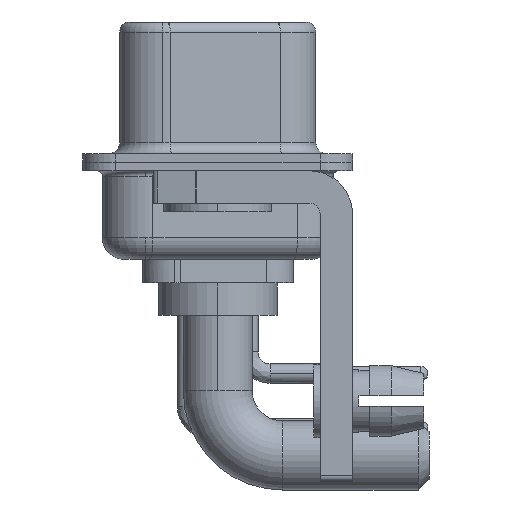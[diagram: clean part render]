
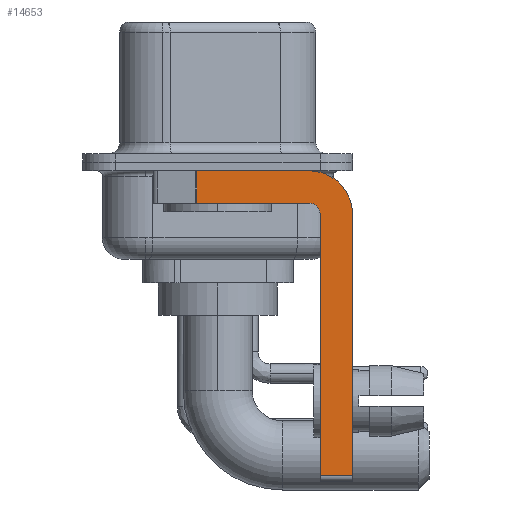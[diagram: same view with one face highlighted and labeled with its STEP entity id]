
A CAD part, left-side view. The second image highlights one B-rep face of the part: STEP entity #14653.
In plain terms, the highlighted planar face has unit normal (-1, 0, 0).
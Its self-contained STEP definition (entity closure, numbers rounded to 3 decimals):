
#846 = DIRECTION ( 'NONE',  ( 0., 0., -1. ) ) ;
#944 = EDGE_CURVE ( 'NONE', #23648, #19559, #24947, .T. ) ;
#1012 = VERTEX_POINT ( 'NONE', #1270 ) ;
#1270 = CARTESIAN_POINT ( 'NONE',  ( -2.9, -4.25, -0.4 ) ) ;
#1272 = LINE ( 'NONE', #3926, #5003 ) ;
#1379 = CARTESIAN_POINT ( 'NONE',  ( -2.9, 3., -0.4 ) ) ;
#2157 = VECTOR ( 'NONE', #846, 1000. ) ;
#2641 = VECTOR ( 'NONE', #6924, 1000. ) ;
#2652 = ORIENTED_EDGE ( 'NONE', *, *, #17154, .F. ) ;
#3075 = AXIS2_PLACEMENT_3D ( 'NONE', #25043, #11268, #29862 ) ;
#3139 = DIRECTION ( 'NONE',  ( 0., 0., -1. ) ) ;
#3926 = CARTESIAN_POINT ( 'NONE',  ( -2.9, -4.75, -14.8 ) ) ;
#4272 = EDGE_CURVE ( 'NONE', #19559, #4273, #13885, .T. ) ;
#4273 = VERTEX_POINT ( 'NONE', #29976 ) ;
#4449 = AXIS2_PLACEMENT_3D ( 'NONE', #12879, #17130, #22141 ) ;
#5003 = VECTOR ( 'NONE', #8788, 1000. ) ;
#5857 = CARTESIAN_POINT ( 'NONE',  ( -2.9, -4.25, -14.55 ) ) ;
#5903 = EDGE_CURVE ( 'NONE', #22991, #4273, #27285, .T. ) ;
#6349 = EDGE_CURVE ( 'NONE', #22991, #1012, #22850, .T. ) ;
#6483 = DIRECTION ( 'NONE',  ( 1., 0., 0. ) ) ;
#6924 = DIRECTION ( 'NONE',  ( 0., -1., 0. ) ) ;
#7840 = CIRCLE ( 'NONE', #25843, 2. ) ;
#8675 = CARTESIAN_POINT ( 'NONE',  ( -2.9, -6.25, -2.4 ) ) ;
#8788 = DIRECTION ( 'NONE',  ( 0., 0., 1. ) ) ;
#9100 = EDGE_LOOP ( 'NONE', ( #12794, #27243, #21199, #10554, #2652, #26335, #9128, #10559 ) ) ;
#9128 = ORIENTED_EDGE ( 'NONE', *, *, #29358, .F. ) ;
#9729 = LINE ( 'NONE', #28971, #23791 ) ;
#10554 = ORIENTED_EDGE ( 'NONE', *, *, #944, .F. ) ;
#10559 = ORIENTED_EDGE ( 'NONE', *, *, #30675, .F. ) ;
#11067 = CARTESIAN_POINT ( 'NONE',  ( -2.9, -4.25, -1.9 ) ) ;
#11268 = DIRECTION ( 'NONE',  ( 1., 0., 0. ) ) ;
#12794 = ORIENTED_EDGE ( 'NONE', *, *, #6349, .F. ) ;
#12879 = CARTESIAN_POINT ( 'NONE',  ( -2.9, -4.25, -2.4 ) ) ;
#13539 = CARTESIAN_POINT ( 'NONE',  ( -2.9, -4.75, -2.4 ) ) ;
#13574 = DIRECTION ( 'NONE',  ( 0., 1., 0. ) ) ;
#13885 = LINE ( 'NONE', #11067, #28058 ) ;
#14653 = ADVANCED_FACE ( 'NONE', ( #23173 ), #17850, .F. ) ;
#15641 = DIRECTION ( 'NONE',  ( 0., -1., 0. ) ) ;
#15690 = VECTOR ( 'NONE', #15641, 1000. ) ;
#17130 = DIRECTION ( 'NONE',  ( -1., 0., 0. ) ) ;
#17154 = EDGE_CURVE ( 'NONE', #22116, #23648, #1272, .T. ) ;
#17850 = PLANE ( 'NONE',  #3075 ) ;
#18411 = CARTESIAN_POINT ( 'NONE',  ( -2.9, -4.25, -2.4 ) ) ;
#19559 = VERTEX_POINT ( 'NONE', #28901 ) ;
#19721 = EDGE_CURVE ( 'NONE', #22116, #24093, #27313, .T. ) ;
#21071 = DIRECTION ( 'NONE',  ( 0., 0., -1. ) ) ;
#21199 = ORIENTED_EDGE ( 'NONE', *, *, #4272, .F. ) ;
#22116 = VERTEX_POINT ( 'NONE', #24812 ) ;
#22141 = DIRECTION ( 'NONE',  ( 0., 0., 1. ) ) ;
#22497 = CARTESIAN_POINT ( 'NONE',  ( -2.9, 0.978, -0.4 ) ) ;
#22763 = CARTESIAN_POINT ( 'NONE',  ( -2.9, 0.978, -1.9 ) ) ;
#22850 = LINE ( 'NONE', #1379, #15690 ) ;
#22991 = VERTEX_POINT ( 'NONE', #22497 ) ;
#23109 = CARTESIAN_POINT ( 'NONE',  ( -2.9, -6.25, -14.55 ) ) ;
#23173 = FACE_OUTER_BOUND ( 'NONE', #9100, .T. ) ;
#23648 = VERTEX_POINT ( 'NONE', #13539 ) ;
#23791 = VECTOR ( 'NONE', #3139, 1000. ) ;
#24093 = VERTEX_POINT ( 'NONE', #23109 ) ;
#24146 = VERTEX_POINT ( 'NONE', #8675 ) ;
#24812 = CARTESIAN_POINT ( 'NONE',  ( -2.9, -4.75, -14.55 ) ) ;
#24947 = CIRCLE ( 'NONE', #4449, 0.5 ) ;
#25043 = CARTESIAN_POINT ( 'NONE',  ( -2.9, -4.25, -2.4 ) ) ;
#25843 = AXIS2_PLACEMENT_3D ( 'NONE', #18411, #6483, #21071 ) ;
#26335 = ORIENTED_EDGE ( 'NONE', *, *, #19721, .T. ) ;
#27243 = ORIENTED_EDGE ( 'NONE', *, *, #5903, .T. ) ;
#27285 = LINE ( 'NONE', #22763, #2157 ) ;
#27313 = LINE ( 'NONE', #5857, #2641 ) ;
#28058 = VECTOR ( 'NONE', #13574, 1000. ) ;
#28901 = CARTESIAN_POINT ( 'NONE',  ( -2.9, -4.25, -1.9 ) ) ;
#28971 = CARTESIAN_POINT ( 'NONE',  ( -2.9, -6.25, -2.4 ) ) ;
#29358 = EDGE_CURVE ( 'NONE', #24146, #24093, #9729, .T. ) ;
#29862 = DIRECTION ( 'NONE',  ( 0., 0., -1. ) ) ;
#29976 = CARTESIAN_POINT ( 'NONE',  ( -2.9, 0.978, -1.9 ) ) ;
#30675 = EDGE_CURVE ( 'NONE', #1012, #24146, #7840, .T. ) ;
